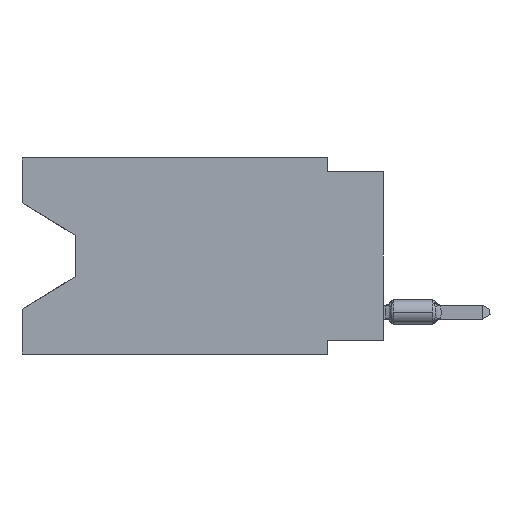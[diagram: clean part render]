
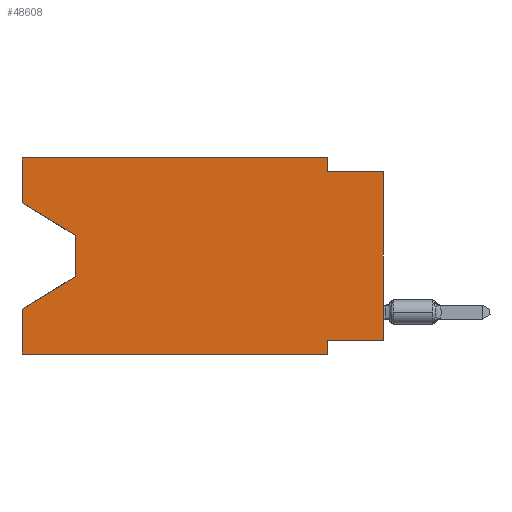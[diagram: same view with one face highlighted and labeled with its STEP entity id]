
A CAD part, left-side view. The second image highlights one B-rep face of the part: STEP entity #48608.
In plain terms, the highlighted planar face has unit normal (-1, 0, 0).
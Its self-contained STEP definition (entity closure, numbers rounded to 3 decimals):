
#1747 = VERTEX_POINT ( 'NONE', #40443 ) ;
#1989 = VECTOR ( 'NONE', #12656, 1000. ) ;
#3837 = CARTESIAN_POINT ( 'NONE',  ( 0., 13.97, -3.505 ) ) ;
#4676 = VERTEX_POINT ( 'NONE', #5569 ) ;
#5569 = CARTESIAN_POINT ( 'NONE',  ( 0., 0., -8.255 ) ) ;
#6602 = LINE ( 'NONE', #16532, #18043 ) ;
#6854 = EDGE_CURVE ( 'NONE', #59014, #46978, #11121, .T. ) ;
#7865 = LINE ( 'NONE', #51124, #29874 ) ;
#8110 = VECTOR ( 'NONE', #57359, 1000. ) ;
#9370 = CARTESIAN_POINT ( 'NONE',  ( 0., 16.383, -2.038 ) ) ;
#9506 = EDGE_CURVE ( 'NONE', #1747, #15331, #19331, .T. ) ;
#9975 = LINE ( 'NONE', #29559, #58116 ) ;
#11121 = LINE ( 'NONE', #40954, #43662 ) ;
#11227 = VERTEX_POINT ( 'NONE', #32471 ) ;
#12223 = VERTEX_POINT ( 'NONE', #57579 ) ;
#12656 = DIRECTION ( 'NONE',  ( 0., 1., 0. ) ) ;
#13196 = DIRECTION ( 'NONE',  ( 0., 0., 1. ) ) ;
#13433 = DIRECTION ( 'NONE',  ( 0., 0., -1. ) ) ;
#13862 = DIRECTION ( 'NONE',  ( 0., -1., 0. ) ) ;
#14749 = CARTESIAN_POINT ( 'NONE',  ( 0., 16.383, 0. ) ) ;
#15331 = VERTEX_POINT ( 'NONE', #51646 ) ;
#15551 = CARTESIAN_POINT ( 'NONE',  ( 0., 2.54, 0. ) ) ;
#15916 = VECTOR ( 'NONE', #42243, 1000. ) ;
#15938 = VERTEX_POINT ( 'NONE', #52282 ) ;
#16532 = CARTESIAN_POINT ( 'NONE',  ( 0., 13.97, -5.385 ) ) ;
#17293 = CARTESIAN_POINT ( 'NONE',  ( 0., 16.383, 0. ) ) ;
#17564 = LINE ( 'NONE', #21752, #15916 ) ;
#18043 = VECTOR ( 'NONE', #56219, 1000. ) ;
#18075 = DIRECTION ( 'NONE',  ( 0., 0., -1. ) ) ;
#19331 = LINE ( 'NONE', #28008, #26475 ) ;
#21752 = CARTESIAN_POINT ( 'NONE',  ( 0., 16.383, -2.038 ) ) ;
#21963 = LINE ( 'NONE', #41499, #58229 ) ;
#22692 = AXIS2_PLACEMENT_3D ( 'NONE', #23538, #37016, #18075 ) ;
#22760 = ORIENTED_EDGE ( 'NONE', *, *, #59029, .F. ) ;
#23538 = CARTESIAN_POINT ( 'NONE',  ( 0., 16.383, 0. ) ) ;
#23790 = EDGE_CURVE ( 'NONE', #1747, #15938, #37576, .T. ) ;
#24103 = VERTEX_POINT ( 'NONE', #43616 ) ;
#24374 = LINE ( 'NONE', #14749, #8110 ) ;
#25421 = VECTOR ( 'NONE', #36056, 1000. ) ;
#26128 = VERTEX_POINT ( 'NONE', #51706 ) ;
#26475 = VECTOR ( 'NONE', #13862, 1000. ) ;
#26698 = ORIENTED_EDGE ( 'NONE', *, *, #58312, .F. ) ;
#28008 = CARTESIAN_POINT ( 'NONE',  ( 0., 16.383, -8.89 ) ) ;
#28061 = CARTESIAN_POINT ( 'NONE',  ( 0., 0., -8.255 ) ) ;
#28555 = ORIENTED_EDGE ( 'NONE', *, *, #39868, .T. ) ;
#29559 = CARTESIAN_POINT ( 'NONE',  ( 0., 2.54, -8.89 ) ) ;
#29874 = VECTOR ( 'NONE', #46634, 1000. ) ;
#30021 = ORIENTED_EDGE ( 'NONE', *, *, #46371, .F. ) ;
#30938 = LINE ( 'NONE', #15551, #25421 ) ;
#32191 = FACE_OUTER_BOUND ( 'NONE', #46485, .T. ) ;
#32471 = CARTESIAN_POINT ( 'NONE',  ( 0., 2.54, -0.635 ) ) ;
#33742 = ORIENTED_EDGE ( 'NONE', *, *, #37896, .T. ) ;
#34183 = ORIENTED_EDGE ( 'NONE', *, *, #49056, .T. ) ;
#34683 = DIRECTION ( 'NONE',  ( 0., 0., -1. ) ) ;
#35859 = ORIENTED_EDGE ( 'NONE', *, *, #23790, .F. ) ;
#35926 = VECTOR ( 'NONE', #13433, 1000. ) ;
#36056 = DIRECTION ( 'NONE',  ( 0., 0., -1. ) ) ;
#37016 = DIRECTION ( 'NONE',  ( 1., 0., 0. ) ) ;
#37576 = LINE ( 'NONE', #48350, #51685 ) ;
#37896 = EDGE_CURVE ( 'NONE', #4676, #58998, #7865, .T. ) ;
#39669 = DIRECTION ( 'NONE',  ( 0., 0., 1. ) ) ;
#39868 = EDGE_CURVE ( 'NONE', #59014, #12223, #17564, .T. ) ;
#40443 = CARTESIAN_POINT ( 'NONE',  ( 0., 16.383, -8.89 ) ) ;
#40954 = CARTESIAN_POINT ( 'NONE',  ( 0., 16.383, 0. ) ) ;
#41499 = CARTESIAN_POINT ( 'NONE',  ( 0., 0., -0.635 ) ) ;
#42243 = DIRECTION ( 'NONE',  ( 0., -0.855, -0.519 ) ) ;
#43616 = CARTESIAN_POINT ( 'NONE',  ( 0., 13.97, -5.385 ) ) ;
#43662 = VECTOR ( 'NONE', #39669, 1000. ) ;
#44336 = VERTEX_POINT ( 'NONE', #63233 ) ;
#44781 = ORIENTED_EDGE ( 'NONE', *, *, #57701, .F. ) ;
#46371 = EDGE_CURVE ( 'NONE', #11227, #58998, #21963, .T. ) ;
#46485 = EDGE_LOOP ( 'NONE', ( #28555, #34183, #59544, #35859, #49962, #22760, #55043, #33742, #30021, #44781, #26698, #52702 ) ) ;
#46634 = DIRECTION ( 'NONE',  ( 0., 0., 1. ) ) ;
#46978 = VERTEX_POINT ( 'NONE', #17293 ) ;
#48350 = CARTESIAN_POINT ( 'NONE',  ( 0., 16.383, 0. ) ) ;
#48608 = ADVANCED_FACE ( 'NONE', ( #32191 ), #61943, .F. ) ;
#49056 = EDGE_CURVE ( 'NONE', #12223, #24103, #53140, .T. ) ;
#49962 = ORIENTED_EDGE ( 'NONE', *, *, #9506, .T. ) ;
#51124 = CARTESIAN_POINT ( 'NONE',  ( 0., 0., 0. ) ) ;
#51646 = CARTESIAN_POINT ( 'NONE',  ( 0., 2.54, -8.89 ) ) ;
#51685 = VECTOR ( 'NONE', #13196, 1000. ) ;
#51706 = CARTESIAN_POINT ( 'NONE',  ( 0., 2.54, -8.255 ) ) ;
#52282 = CARTESIAN_POINT ( 'NONE',  ( 0., 16.383, -6.852 ) ) ;
#52702 = ORIENTED_EDGE ( 'NONE', *, *, #6854, .F. ) ;
#53140 = LINE ( 'NONE', #3837, #35926 ) ;
#54980 = EDGE_CURVE ( 'NONE', #24103, #15938, #6602, .T. ) ;
#55043 = ORIENTED_EDGE ( 'NONE', *, *, #59986, .F. ) ;
#56219 = DIRECTION ( 'NONE',  ( 0., 0.855, -0.519 ) ) ;
#57359 = DIRECTION ( 'NONE',  ( 0., -1., 0. ) ) ;
#57579 = CARTESIAN_POINT ( 'NONE',  ( 0., 13.97, -3.505 ) ) ;
#57701 = EDGE_CURVE ( 'NONE', #44336, #11227, #30938, .T. ) ;
#58116 = VECTOR ( 'NONE', #34683, 1000. ) ;
#58229 = VECTOR ( 'NONE', #61000, 1000. ) ;
#58312 = EDGE_CURVE ( 'NONE', #46978, #44336, #24374, .T. ) ;
#58968 = CARTESIAN_POINT ( 'NONE',  ( 0., 0., -0.635 ) ) ;
#58998 = VERTEX_POINT ( 'NONE', #58968 ) ;
#59014 = VERTEX_POINT ( 'NONE', #9370 ) ;
#59029 = EDGE_CURVE ( 'NONE', #26128, #15331, #9975, .T. ) ;
#59544 = ORIENTED_EDGE ( 'NONE', *, *, #54980, .T. ) ;
#59986 = EDGE_CURVE ( 'NONE', #4676, #26128, #62926, .T. ) ;
#61000 = DIRECTION ( 'NONE',  ( 0., -1., 0. ) ) ;
#61943 = PLANE ( 'NONE',  #22692 ) ;
#62926 = LINE ( 'NONE', #28061, #1989 ) ;
#63233 = CARTESIAN_POINT ( 'NONE',  ( 0., 2.54, 0. ) ) ;
